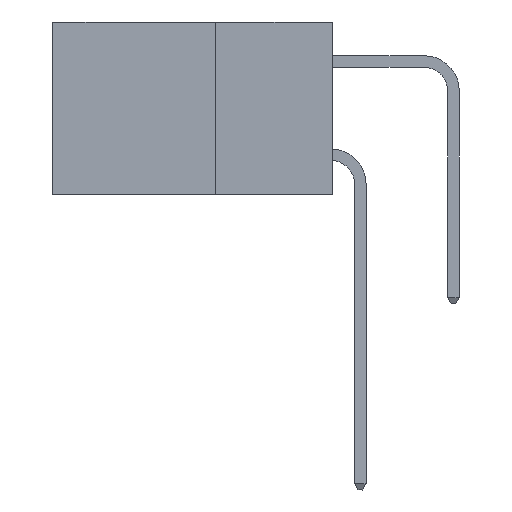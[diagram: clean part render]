
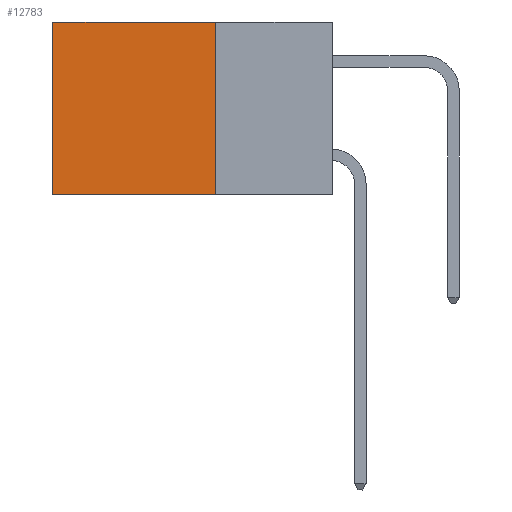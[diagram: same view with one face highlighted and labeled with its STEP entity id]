
A CAD part, left-side view. The second image highlights one B-rep face of the part: STEP entity #12783.
In plain terms, the highlighted planar face has unit normal (-1, 0, 0).
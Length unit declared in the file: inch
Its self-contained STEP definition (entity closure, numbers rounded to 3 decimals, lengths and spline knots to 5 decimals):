
#686 = EDGE_CURVE ( 'NONE', #11292, #11267, #1346, .T. ) ;
#950 = VECTOR ( 'NONE', #11384, 39.37008 ) ;
#1346 = LINE ( 'NONE', #5033, #8197 ) ;
#1855 = FACE_OUTER_BOUND ( 'NONE', #7397, .T. ) ;
#2950 = LINE ( 'NONE', #13398, #6151 ) ;
#3144 = AXIS2_PLACEMENT_3D ( 'NONE', #4866, #6532, #10823 ) ;
#3556 = LINE ( 'NONE', #13289, #9040 ) ;
#3630 = EDGE_CURVE ( 'NONE', #7466, #9407, #2950, .T. ) ;
#4025 = EDGE_CURVE ( 'NONE', #11292, #7466, #10552, .T. ) ;
#4866 = CARTESIAN_POINT ( 'NONE',  ( 0.298, 0.25, 0. ) ) ;
#5033 = CARTESIAN_POINT ( 'NONE',  ( 0.298, 0.25, 0. ) ) ;
#6151 = VECTOR ( 'NONE', #13674, 39.37008 ) ;
#6532 = DIRECTION ( 'NONE',  ( 1., 0., 0. ) ) ;
#6718 = ORIENTED_EDGE ( 'NONE', *, *, #3630, .F. ) ;
#7332 = CARTESIAN_POINT ( 'NONE',  ( 0.298, 0.25, 0. ) ) ;
#7397 = EDGE_LOOP ( 'NONE', ( #8674, #6718, #7565, #11440 ) ) ;
#7466 = VERTEX_POINT ( 'NONE', #13879 ) ;
#7565 = ORIENTED_EDGE ( 'NONE', *, *, #4025, .F. ) ;
#8197 = VECTOR ( 'NONE', #10750, 39.37008 ) ;
#8345 = CARTESIAN_POINT ( 'NONE',  ( 0.298, 0.6, 0. ) ) ;
#8674 = ORIENTED_EDGE ( 'NONE', *, *, #14607, .T. ) ;
#9040 = VECTOR ( 'NONE', #10582, 39.37008 ) ;
#9407 = VERTEX_POINT ( 'NONE', #12410 ) ;
#10552 = LINE ( 'NONE', #7332, #950 ) ;
#10582 = DIRECTION ( 'NONE',  ( 0., 0., -1. ) ) ;
#10750 = DIRECTION ( 'NONE',  ( 0., 1., 0. ) ) ;
#10823 = DIRECTION ( 'NONE',  ( 0., 0., -1. ) ) ;
#11267 = VERTEX_POINT ( 'NONE', #8345 ) ;
#11292 = VERTEX_POINT ( 'NONE', #13787 ) ;
#11384 = DIRECTION ( 'NONE',  ( 0., 0., -1. ) ) ;
#11440 = ORIENTED_EDGE ( 'NONE', *, *, #686, .T. ) ;
#12410 = CARTESIAN_POINT ( 'NONE',  ( 0.298, 0.6, -0.37 ) ) ;
#12783 = ADVANCED_FACE ( 'NONE', ( #1855 ), #15585, .F. ) ;
#13289 = CARTESIAN_POINT ( 'NONE',  ( 0.298, 0.6, 0. ) ) ;
#13398 = CARTESIAN_POINT ( 'NONE',  ( 0.298, 0.25, -0.37 ) ) ;
#13674 = DIRECTION ( 'NONE',  ( 0., 1., 0. ) ) ;
#13787 = CARTESIAN_POINT ( 'NONE',  ( 0.298, 0.25, 0. ) ) ;
#13879 = CARTESIAN_POINT ( 'NONE',  ( 0.298, 0.25, -0.37 ) ) ;
#14607 = EDGE_CURVE ( 'NONE', #11267, #9407, #3556, .T. ) ;
#15585 = PLANE ( 'NONE',  #3144 ) ;
